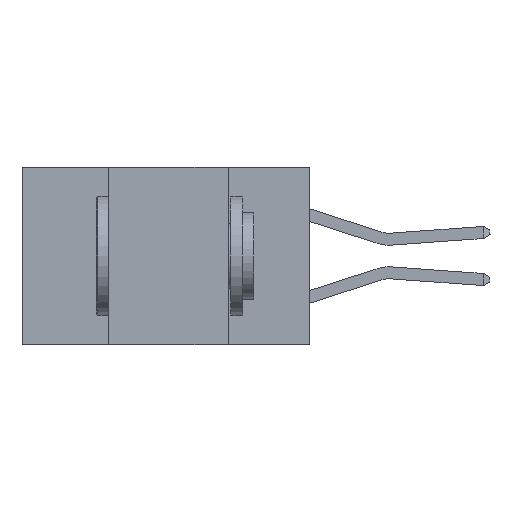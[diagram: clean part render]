
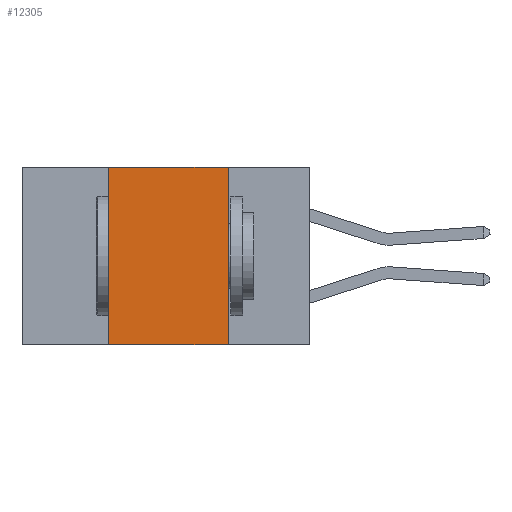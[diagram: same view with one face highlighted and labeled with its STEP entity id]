
A CAD part, left-side view. The second image highlights one B-rep face of the part: STEP entity #12305.
In plain terms, the highlighted planar face has unit normal (-1, 0, 0).
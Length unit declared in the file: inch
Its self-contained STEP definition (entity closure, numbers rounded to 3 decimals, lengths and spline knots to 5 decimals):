
#159 = VERTEX_POINT ( 'NONE', #7223 ) ;
#162 = AXIS2_PLACEMENT_3D ( 'NONE', #4577, #5604, #8571 ) ;
#282 = LINE ( 'NONE', #1285, #4634 ) ;
#385 = CARTESIAN_POINT ( 'NONE',  ( 0., 0.17, -0.37 ) ) ;
#979 = EDGE_CURVE ( 'NONE', #6093, #9417, #282, .T. ) ;
#1086 = VERTEX_POINT ( 'NONE', #4230 ) ;
#1285 = CARTESIAN_POINT ( 'NONE',  ( 0., 0.6, 0. ) ) ;
#1449 = DIRECTION ( 'NONE',  ( 0., 0., -1. ) ) ;
#1496 = FACE_OUTER_BOUND ( 'NONE', #4222, .T. ) ;
#2456 = VECTOR ( 'NONE', #1449, 39.37008 ) ;
#2623 = PLANE ( 'NONE',  #162 ) ;
#2793 = LINE ( 'NONE', #11421, #5247 ) ;
#2822 = CARTESIAN_POINT ( 'NONE',  ( 0., 0.17, 0. ) ) ;
#3117 = ORIENTED_EDGE ( 'NONE', *, *, #8986, .F. ) ;
#3244 = ORIENTED_EDGE ( 'NONE', *, *, #979, .F. ) ;
#4009 = EDGE_CURVE ( 'NONE', #1086, #159, #2793, .T. ) ;
#4037 = CARTESIAN_POINT ( 'NONE',  ( 0., 0.42, 0. ) ) ;
#4222 = EDGE_LOOP ( 'NONE', ( #5375, #3244, #3117, #12564 ) ) ;
#4230 = CARTESIAN_POINT ( 'NONE',  ( 0., 0.42, -0.37 ) ) ;
#4577 = CARTESIAN_POINT ( 'NONE',  ( 0., 0.6, 0. ) ) ;
#4634 = VECTOR ( 'NONE', #11401, 39.37008 ) ;
#4891 = EDGE_CURVE ( 'NONE', #9417, #159, #5358, .T. ) ;
#5247 = VECTOR ( 'NONE', #8749, 39.37008 ) ;
#5358 = LINE ( 'NONE', #385, #2456 ) ;
#5375 = ORIENTED_EDGE ( 'NONE', *, *, #4891, .F. ) ;
#5604 = DIRECTION ( 'NONE',  ( 1., 0., 0. ) ) ;
#6093 = VERTEX_POINT ( 'NONE', #4037 ) ;
#7223 = CARTESIAN_POINT ( 'NONE',  ( 0., 0.17, -0.37 ) ) ;
#8571 = DIRECTION ( 'NONE',  ( 0., 0., -1. ) ) ;
#8749 = DIRECTION ( 'NONE',  ( 0., -1., 0. ) ) ;
#8798 = CARTESIAN_POINT ( 'NONE',  ( 0., 0.42, -0.37 ) ) ;
#8986 = EDGE_CURVE ( 'NONE', #1086, #6093, #10112, .T. ) ;
#9417 = VERTEX_POINT ( 'NONE', #2822 ) ;
#10112 = LINE ( 'NONE', #8798, #11210 ) ;
#11210 = VECTOR ( 'NONE', #11919, 39.37008 ) ;
#11401 = DIRECTION ( 'NONE',  ( 0., -1., 0. ) ) ;
#11421 = CARTESIAN_POINT ( 'NONE',  ( 0., 0.6, -0.37 ) ) ;
#11919 = DIRECTION ( 'NONE',  ( 0., 0., 1. ) ) ;
#12305 = ADVANCED_FACE ( 'NONE', ( #1496 ), #2623, .F. ) ;
#12564 = ORIENTED_EDGE ( 'NONE', *, *, #4009, .T. ) ;
